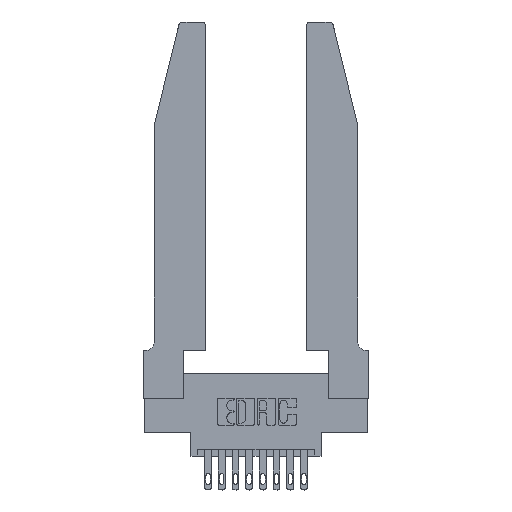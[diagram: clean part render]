
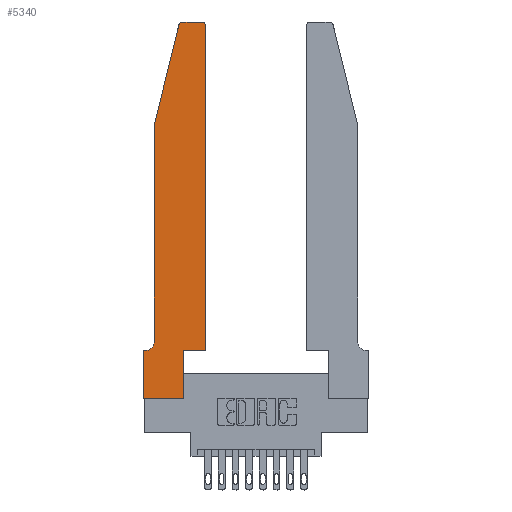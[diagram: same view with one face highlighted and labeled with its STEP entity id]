
A CAD part, top view. The second image highlights one B-rep face of the part: STEP entity #5340.
In plain terms, the highlighted planar face has unit normal (0, 0, 1).
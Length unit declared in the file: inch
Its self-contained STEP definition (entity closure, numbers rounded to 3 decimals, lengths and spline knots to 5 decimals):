
#167 = LINE ( 'NONE', #15054, #4129 ) ;
#282 = AXIS2_PLACEMENT_3D ( 'NONE', #10743, #3297, #15419 ) ;
#374 = VERTEX_POINT ( 'NONE', #5191 ) ;
#452 = ORIENTED_EDGE ( 'NONE', *, *, #2569, .T. ) ;
#605 = CARTESIAN_POINT ( 'NONE',  ( 0.0055, 0.35, 0.37 ) ) ;
#795 = VERTEX_POINT ( 'NONE', #8960 ) ;
#832 = CARTESIAN_POINT ( 'NONE',  ( 0.4505, 0.35, 0.37 ) ) ;
#1028 = DIRECTION ( 'NONE',  ( 0., 0., -1. ) ) ;
#1094 = DIRECTION ( 'NONE',  ( 0., 0., 1. ) ) ;
#1242 = DIRECTION ( 'NONE',  ( 0., -1., 0. ) ) ;
#1425 = ORIENTED_EDGE ( 'NONE', *, *, #3678, .T. ) ;
#1585 = PLANE ( 'NONE',  #7834 ) ;
#1670 = EDGE_LOOP ( 'NONE', ( #1425, #5545, #5114, #14263, #13923, #3234, #5031, #5904, #452, #11825, #4537, #10694 ) ) ;
#1702 = CIRCLE ( 'NONE', #9873, 0.03 ) ;
#1753 = CARTESIAN_POINT ( 'NONE',  ( 0., 0., 0.37 ) ) ;
#1907 = EDGE_CURVE ( 'NONE', #11069, #4475, #1702, .T. ) ;
#2110 = CARTESIAN_POINT ( 'NONE',  ( 0.4205, 2.75, 0.37 ) ) ;
#2194 = LINE ( 'NONE', #8249, #9765 ) ;
#2569 = EDGE_CURVE ( 'NONE', #374, #3446, #167, .T. ) ;
#2780 = VERTEX_POINT ( 'NONE', #12914 ) ;
#2795 = LINE ( 'NONE', #15576, #11126 ) ;
#2934 = LINE ( 'NONE', #1753, #15252 ) ;
#3234 = ORIENTED_EDGE ( 'NONE', *, *, #5188, .T. ) ;
#3297 = DIRECTION ( 'NONE',  ( 0., 0., 1. ) ) ;
#3304 = EDGE_CURVE ( 'NONE', #14673, #795, #2795, .T. ) ;
#3369 = VECTOR ( 'NONE', #10882, 39.37008 ) ;
#3446 = VERTEX_POINT ( 'NONE', #14459 ) ;
#3678 = EDGE_CURVE ( 'NONE', #4475, #11487, #10542, .T. ) ;
#3936 = DIRECTION ( 'NONE',  ( 0., 1., 0. ) ) ;
#3988 = CARTESIAN_POINT ( 'NONE',  ( 0.4505, 0.35, 0.37 ) ) ;
#4129 = VECTOR ( 'NONE', #15153, 39.37008 ) ;
#4440 = LINE ( 'NONE', #14527, #14513 ) ;
#4475 = VERTEX_POINT ( 'NONE', #2110 ) ;
#4537 = ORIENTED_EDGE ( 'NONE', *, *, #9064, .T. ) ;
#4571 = DIRECTION ( 'NONE',  ( 1., 0., 0. ) ) ;
#4961 = EDGE_CURVE ( 'NONE', #795, #8946, #4440, .T. ) ;
#4962 = EDGE_CURVE ( 'NONE', #11648, #6821, #2194, .T. ) ;
#5031 = ORIENTED_EDGE ( 'NONE', *, *, #4962, .T. ) ;
#5098 = VECTOR ( 'NONE', #3936, 39.37008 ) ;
#5114 = ORIENTED_EDGE ( 'NONE', *, *, #3304, .T. ) ;
#5188 = EDGE_CURVE ( 'NONE', #13027, #11648, #11872, .T. ) ;
#5191 = CARTESIAN_POINT ( 'NONE',  ( 0.2865, 0., 0.37 ) ) ;
#5337 = EDGE_CURVE ( 'NONE', #6821, #374, #2934, .T. ) ;
#5340 = ADVANCED_FACE ( 'NONE', ( #9933 ), #1585, .T. ) ;
#5363 = DIRECTION ( 'NONE',  ( 0., 0., 1. ) ) ;
#5545 = ORIENTED_EDGE ( 'NONE', *, *, #8394, .T. ) ;
#5817 = CARTESIAN_POINT ( 'NONE',  ( 0.0755, 0.35, 0.37 ) ) ;
#5904 = ORIENTED_EDGE ( 'NONE', *, *, #5337, .T. ) ;
#6340 = CARTESIAN_POINT ( 'NONE',  ( 0.4505, 2.72, 0.37 ) ) ;
#6376 = DIRECTION ( 'NONE',  ( 1., 0., 0. ) ) ;
#6821 = VERTEX_POINT ( 'NONE', #10427 ) ;
#7262 = DIRECTION ( 'NONE',  ( 0., -1., 0. ) ) ;
#7834 = AXIS2_PLACEMENT_3D ( 'NONE', #12655, #5363, #13865 ) ;
#8049 = DIRECTION ( 'NONE',  ( -1., 0., 0. ) ) ;
#8144 = EDGE_CURVE ( 'NONE', #3446, #2780, #13298, .T. ) ;
#8249 = CARTESIAN_POINT ( 'NONE',  ( 0., 0., 0.37 ) ) ;
#8348 = CIRCLE ( 'NONE', #282, 0.03 ) ;
#8394 = EDGE_CURVE ( 'NONE', #11487, #14673, #8348, .T. ) ;
#8757 = CARTESIAN_POINT ( 'NONE',  ( 0.25487, 2.72718, 0.37 ) ) ;
#8946 = VERTEX_POINT ( 'NONE', #9030 ) ;
#8960 = CARTESIAN_POINT ( 'NONE',  ( 0.0755, 2., 0.37 ) ) ;
#9030 = CARTESIAN_POINT ( 'NONE',  ( 0.0755, 0.42, 0.37 ) ) ;
#9064 = EDGE_CURVE ( 'NONE', #2780, #11069, #14793, .T. ) ;
#9108 = EDGE_CURVE ( 'NONE', #8946, #13027, #10790, .T. ) ;
#9645 = AXIS2_PLACEMENT_3D ( 'NONE', #10648, #1028, #11914 ) ;
#9690 = CARTESIAN_POINT ( 'NONE',  ( 0.2605, 2.75, 0.37 ) ) ;
#9765 = VECTOR ( 'NONE', #1242, 39.37008 ) ;
#9873 = AXIS2_PLACEMENT_3D ( 'NONE', #11868, #1094, #4571 ) ;
#9933 = FACE_OUTER_BOUND ( 'NONE', #1670, .T. ) ;
#10132 = VECTOR ( 'NONE', #8049, 39.37008 ) ;
#10418 = DIRECTION ( 'NONE',  ( 1., 0., 0. ) ) ;
#10427 = CARTESIAN_POINT ( 'NONE',  ( 0., 0., 0.37 ) ) ;
#10542 = LINE ( 'NONE', #9690, #3369 ) ;
#10578 = DIRECTION ( 'NONE',  ( -0.239, -0.971, 0. ) ) ;
#10648 = CARTESIAN_POINT ( 'NONE',  ( 0.0055, 0.42, 0.37 ) ) ;
#10694 = ORIENTED_EDGE ( 'NONE', *, *, #1907, .T. ) ;
#10743 = CARTESIAN_POINT ( 'NONE',  ( 0.284, 2.72, 0.37 ) ) ;
#10790 = CIRCLE ( 'NONE', #9645, 0.07 ) ;
#10882 = DIRECTION ( 'NONE',  ( -1., 0., 0. ) ) ;
#11069 = VERTEX_POINT ( 'NONE', #6340 ) ;
#11126 = VECTOR ( 'NONE', #10578, 39.37008 ) ;
#11487 = VERTEX_POINT ( 'NONE', #13769 ) ;
#11606 = CARTESIAN_POINT ( 'NONE',  ( 0., 0.35, 0.37 ) ) ;
#11648 = VERTEX_POINT ( 'NONE', #11606 ) ;
#11825 = ORIENTED_EDGE ( 'NONE', *, *, #8144, .T. ) ;
#11868 = CARTESIAN_POINT ( 'NONE',  ( 0.4205, 2.72, 0.37 ) ) ;
#11872 = LINE ( 'NONE', #5817, #10132 ) ;
#11914 = DIRECTION ( 'NONE',  ( -1., 0., 0. ) ) ;
#12655 = CARTESIAN_POINT ( 'NONE',  ( 0., 0.35, 0.37 ) ) ;
#12914 = CARTESIAN_POINT ( 'NONE',  ( 0.4505, 0.35, 0.37 ) ) ;
#13027 = VERTEX_POINT ( 'NONE', #605 ) ;
#13298 = LINE ( 'NONE', #832, #14629 ) ;
#13769 = CARTESIAN_POINT ( 'NONE',  ( 0.284, 2.75, 0.37 ) ) ;
#13865 = DIRECTION ( 'NONE',  ( 1., 0., 0. ) ) ;
#13923 = ORIENTED_EDGE ( 'NONE', *, *, #9108, .T. ) ;
#14263 = ORIENTED_EDGE ( 'NONE', *, *, #4961, .T. ) ;
#14459 = CARTESIAN_POINT ( 'NONE',  ( 0.2865, 0.35, 0.37 ) ) ;
#14513 = VECTOR ( 'NONE', #7262, 39.37008 ) ;
#14527 = CARTESIAN_POINT ( 'NONE',  ( 0.0755, 2., 0.37 ) ) ;
#14629 = VECTOR ( 'NONE', #10418, 39.37008 ) ;
#14673 = VERTEX_POINT ( 'NONE', #8757 ) ;
#14793 = LINE ( 'NONE', #3988, #5098 ) ;
#15054 = CARTESIAN_POINT ( 'NONE',  ( 0.2865, 0.35, 0.37 ) ) ;
#15153 = DIRECTION ( 'NONE',  ( 0., 1., 0. ) ) ;
#15252 = VECTOR ( 'NONE', #6376, 39.37008 ) ;
#15419 = DIRECTION ( 'NONE',  ( 1., 0., 0. ) ) ;
#15576 = CARTESIAN_POINT ( 'NONE',  ( 0.0755, 2., 0.37 ) ) ;
